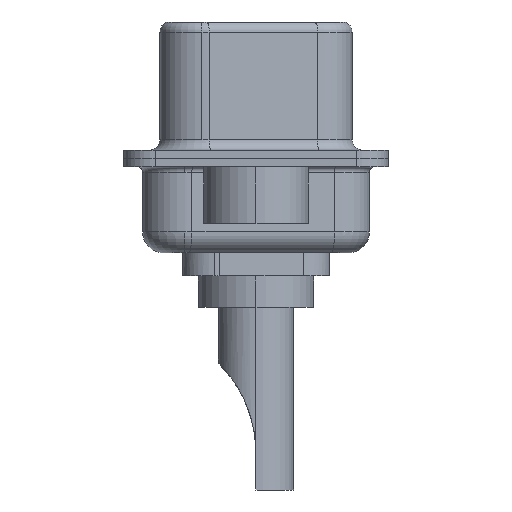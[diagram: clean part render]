
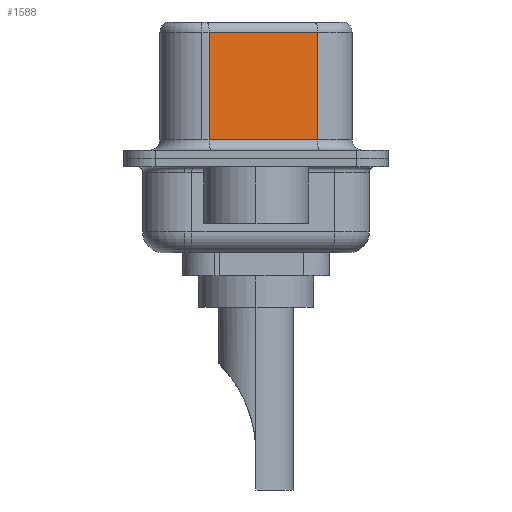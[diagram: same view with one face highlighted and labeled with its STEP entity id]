
A CAD part, left-side view. The second image highlights one B-rep face of the part: STEP entity #1588.
In plain terms, the highlighted planar face has unit normal (-0.985, -0.174, 0).
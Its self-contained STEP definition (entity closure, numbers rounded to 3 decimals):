
#242 = VECTOR ( 'NONE', #6261, 1000. ) ;
#1105 = CARTESIAN_POINT ( 'NONE',  ( 3.675, 2.233, 6.02 ) ) ;
#1588 = ADVANCED_FACE ( 'NONE', ( #5837 ), #9024, .F. ) ;
#1592 = EDGE_LOOP ( 'NONE', ( #3137, #6790, #5324, #7641 ) ) ;
#2106 = DIRECTION ( 'NONE',  ( 0.174, -0.985, 0. ) ) ;
#3137 = ORIENTED_EDGE ( 'NONE', *, *, #3420, .F. ) ;
#3420 = EDGE_CURVE ( 'NONE', #7330, #16415, #16451, .T. ) ;
#5324 = ORIENTED_EDGE ( 'NONE', *, *, #11716, .T. ) ;
#5818 = VERTEX_POINT ( 'NONE', #17084 ) ;
#5837 = FACE_OUTER_BOUND ( 'NONE', #1592, .T. ) ;
#6261 = DIRECTION ( 'NONE',  ( -0.174, 0.985, 0. ) ) ;
#6740 = VECTOR ( 'NONE', #2106, 1000. ) ;
#6790 = ORIENTED_EDGE ( 'NONE', *, *, #10344, .T. ) ;
#7253 = CARTESIAN_POINT ( 'NONE',  ( 3.675, 2.233, 6.52 ) ) ;
#7330 = VERTEX_POINT ( 'NONE', #16785 ) ;
#7369 = EDGE_CURVE ( 'NONE', #5818, #16415, #13871, .T. ) ;
#7641 = ORIENTED_EDGE ( 'NONE', *, *, #7369, .T. ) ;
#8052 = CARTESIAN_POINT ( 'NONE',  ( 4.585, -2.927, 0.9 ) ) ;
#8190 = CARTESIAN_POINT ( 'NONE',  ( 4.585, -2.927, 6.52 ) ) ;
#8445 = VECTOR ( 'NONE', #15268, 1000. ) ;
#9024 = PLANE ( 'NONE',  #12061 ) ;
#10344 = EDGE_CURVE ( 'NONE', #7330, #11236, #10991, .T. ) ;
#10991 = LINE ( 'NONE', #11611, #242 ) ;
#11236 = VERTEX_POINT ( 'NONE', #1105 ) ;
#11585 = CARTESIAN_POINT ( 'NONE',  ( 4.585, -2.927, 0.9 ) ) ;
#11611 = CARTESIAN_POINT ( 'NONE',  ( 4.585, -2.927, 6.02 ) ) ;
#11716 = EDGE_CURVE ( 'NONE', #11236, #5818, #14641, .T. ) ;
#12061 = AXIS2_PLACEMENT_3D ( 'NONE', #8190, #16977, #15556 ) ;
#12776 = DIRECTION ( 'NONE',  ( 0., 0., -1. ) ) ;
#12966 = VECTOR ( 'NONE', #12776, 1000. ) ;
#13354 = CARTESIAN_POINT ( 'NONE',  ( 4.585, -2.927, 6.52 ) ) ;
#13871 = LINE ( 'NONE', #11585, #6740 ) ;
#14641 = LINE ( 'NONE', #7253, #8445 ) ;
#15268 = DIRECTION ( 'NONE',  ( 0., 0., -1. ) ) ;
#15556 = DIRECTION ( 'NONE',  ( -0.174, 0.985, 0. ) ) ;
#16415 = VERTEX_POINT ( 'NONE', #8052 ) ;
#16451 = LINE ( 'NONE', #13354, #12966 ) ;
#16785 = CARTESIAN_POINT ( 'NONE',  ( 4.585, -2.927, 6.02 ) ) ;
#16977 = DIRECTION ( 'NONE',  ( 0.985, 0.174, 0. ) ) ;
#17084 = CARTESIAN_POINT ( 'NONE',  ( 3.675, 2.233, 0.9 ) ) ;
